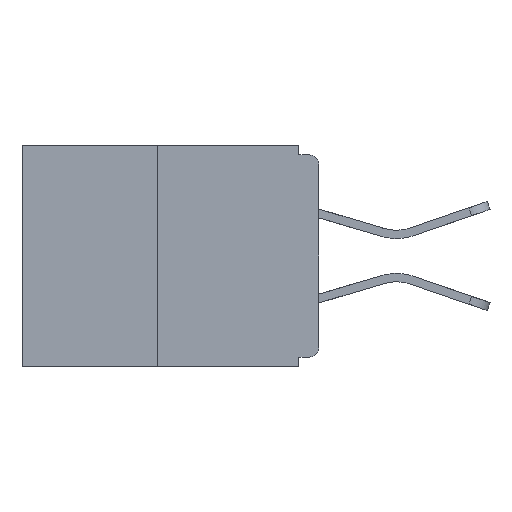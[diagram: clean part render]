
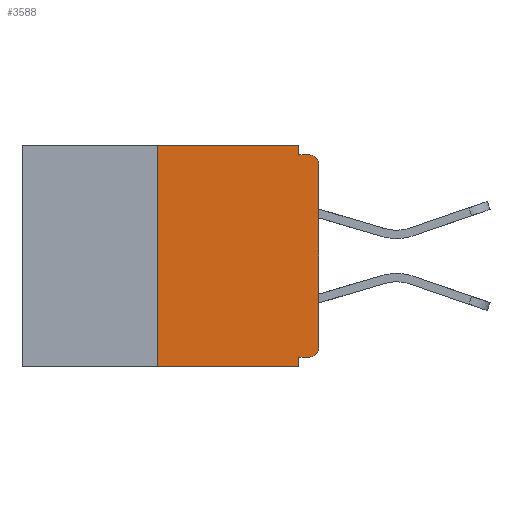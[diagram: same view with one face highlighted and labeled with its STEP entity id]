
A CAD part, left-side view. The second image highlights one B-rep face of the part: STEP entity #3588.
In plain terms, the highlighted planar face has unit normal (-1, 0, 0).
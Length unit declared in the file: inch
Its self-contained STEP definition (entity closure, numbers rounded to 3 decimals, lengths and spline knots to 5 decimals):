
#286 = VERTEX_POINT ( 'NONE', #1986 ) ;
#363 = DIRECTION ( 'NONE',  ( 0., -1., 0. ) ) ;
#559 = CARTESIAN_POINT ( 'NONE',  ( 0., 0.25, 0. ) ) ;
#690 = CARTESIAN_POINT ( 'NONE',  ( 0., 0.46, 0. ) ) ;
#737 = PLANE ( 'NONE',  #10381 ) ;
#957 = ORIENTED_EDGE ( 'NONE', *, *, #11185, .T. ) ;
#1065 = LINE ( 'NONE', #8605, #7907 ) ;
#1281 = CARTESIAN_POINT ( 'NONE',  ( 0., 0.015, -0.015 ) ) ;
#1345 = CARTESIAN_POINT ( 'NONE',  ( 0., 0.015, -0.03 ) ) ;
#1426 = VECTOR ( 'NONE', #13234, 39.37008 ) ;
#1463 = DIRECTION ( 'NONE',  ( 0., -1., 0. ) ) ;
#1663 = LINE ( 'NONE', #2857, #1981 ) ;
#1704 = ORIENTED_EDGE ( 'NONE', *, *, #7658, .T. ) ;
#1903 = VECTOR ( 'NONE', #12912, 39.37008 ) ;
#1948 = CARTESIAN_POINT ( 'NONE',  ( 0., 0., -0.313 ) ) ;
#1981 = VECTOR ( 'NONE', #12138, 39.37008 ) ;
#1986 = CARTESIAN_POINT ( 'NONE',  ( 0., 0.031, -0.015 ) ) ;
#2129 = EDGE_CURVE ( 'NONE', #10455, #8525, #2821, .T. ) ;
#2291 = EDGE_CURVE ( 'NONE', #10760, #11855, #3197, .T. ) ;
#2369 = VERTEX_POINT ( 'NONE', #13059 ) ;
#2490 = ORIENTED_EDGE ( 'NONE', *, *, #3497, .F. ) ;
#2585 = EDGE_LOOP ( 'NONE', ( #2795, #2490, #1704, #7091, #9048, #3241, #957, #9524, #6849, #12381 ) ) ;
#2738 = VERTEX_POINT ( 'NONE', #6238 ) ;
#2795 = ORIENTED_EDGE ( 'NONE', *, *, #9120, .F. ) ;
#2821 = CIRCLE ( 'NONE', #9344, 0.015 ) ;
#2857 = CARTESIAN_POINT ( 'NONE',  ( 0., 0., 0. ) ) ;
#3197 = CIRCLE ( 'NONE', #6318, 0.015 ) ;
#3241 = ORIENTED_EDGE ( 'NONE', *, *, #2291, .T. ) ;
#3264 = EDGE_CURVE ( 'NONE', #2369, #286, #12860, .T. ) ;
#3497 = EDGE_CURVE ( 'NONE', #11511, #11041, #5757, .T. ) ;
#3550 = LINE ( 'NONE', #11971, #1903 ) ;
#3588 = ADVANCED_FACE ( 'NONE', ( #9647 ), #737, .F. ) ;
#3921 = CARTESIAN_POINT ( 'NONE',  ( 0., 0., -0.03 ) ) ;
#3996 = CARTESIAN_POINT ( 'NONE',  ( 0., 0., -0.328 ) ) ;
#4006 = DIRECTION ( 'NONE',  ( 0., 0., -1. ) ) ;
#4123 = VECTOR ( 'NONE', #11197, 39.37008 ) ;
#4186 = DIRECTION ( 'NONE',  ( 0., 0., -1. ) ) ;
#4202 = LINE ( 'NONE', #11248, #1426 ) ;
#4496 = DIRECTION ( 'NONE',  ( -1., 0., 0. ) ) ;
#5285 = CARTESIAN_POINT ( 'NONE',  ( 0., 0.25, -0.343 ) ) ;
#5757 = LINE ( 'NONE', #559, #11089 ) ;
#5895 = DIRECTION ( 'NONE',  ( 0., 0., -1. ) ) ;
#6238 = CARTESIAN_POINT ( 'NONE',  ( 0., 0.031, -0.328 ) ) ;
#6318 = AXIS2_PLACEMENT_3D ( 'NONE', #10951, #9911, #5895 ) ;
#6636 = CARTESIAN_POINT ( 'NONE',  ( 0., 0.031, -0.343 ) ) ;
#6849 = ORIENTED_EDGE ( 'NONE', *, *, #12982, .F. ) ;
#7091 = ORIENTED_EDGE ( 'NONE', *, *, #7758, .F. ) ;
#7441 = DIRECTION ( 'NONE',  ( 0., 0., -1. ) ) ;
#7658 = EDGE_CURVE ( 'NONE', #11511, #11618, #3550, .T. ) ;
#7684 = CARTESIAN_POINT ( 'NONE',  ( 0., 0.25, 0. ) ) ;
#7758 = EDGE_CURVE ( 'NONE', #2738, #11618, #4202, .T. ) ;
#7787 = LINE ( 'NONE', #10745, #8442 ) ;
#7837 = DIRECTION ( 'NONE',  ( 0., 0., 1. ) ) ;
#7907 = VECTOR ( 'NONE', #363, 39.37008 ) ;
#8023 = DIRECTION ( 'NONE',  ( 1., 0., 0. ) ) ;
#8032 = VECTOR ( 'NONE', #4186, 39.37008 ) ;
#8442 = VECTOR ( 'NONE', #1463, 39.37008 ) ;
#8525 = VERTEX_POINT ( 'NONE', #1281 ) ;
#8605 = CARTESIAN_POINT ( 'NONE',  ( 0., 0.46, 0. ) ) ;
#8828 = CARTESIAN_POINT ( 'NONE',  ( 0., 0.015, -0.328 ) ) ;
#9048 = ORIENTED_EDGE ( 'NONE', *, *, #11249, .F. ) ;
#9120 = EDGE_CURVE ( 'NONE', #11041, #2369, #1065, .T. ) ;
#9344 = AXIS2_PLACEMENT_3D ( 'NONE', #1345, #4496, #7441 ) ;
#9524 = ORIENTED_EDGE ( 'NONE', *, *, #2129, .T. ) ;
#9563 = CARTESIAN_POINT ( 'NONE',  ( 0., 0.031, 0. ) ) ;
#9647 = FACE_OUTER_BOUND ( 'NONE', #2585, .T. ) ;
#9911 = DIRECTION ( 'NONE',  ( -1., 0., 0. ) ) ;
#10381 = AXIS2_PLACEMENT_3D ( 'NONE', #690, #8023, #4006 ) ;
#10455 = VERTEX_POINT ( 'NONE', #3921 ) ;
#10745 = CARTESIAN_POINT ( 'NONE',  ( 0., 0., -0.015 ) ) ;
#10760 = VERTEX_POINT ( 'NONE', #8828 ) ;
#10951 = CARTESIAN_POINT ( 'NONE',  ( 0., 0.015, -0.313 ) ) ;
#11041 = VERTEX_POINT ( 'NONE', #7684 ) ;
#11089 = VECTOR ( 'NONE', #7837, 39.37008 ) ;
#11185 = EDGE_CURVE ( 'NONE', #11855, #10455, #1663, .T. ) ;
#11197 = DIRECTION ( 'NONE',  ( 0., 1., 0. ) ) ;
#11217 = LINE ( 'NONE', #3996, #4123 ) ;
#11248 = CARTESIAN_POINT ( 'NONE',  ( 0., 0.031, -0.343 ) ) ;
#11249 = EDGE_CURVE ( 'NONE', #10760, #2738, #11217, .T. ) ;
#11511 = VERTEX_POINT ( 'NONE', #5285 ) ;
#11618 = VERTEX_POINT ( 'NONE', #6636 ) ;
#11855 = VERTEX_POINT ( 'NONE', #1948 ) ;
#11971 = CARTESIAN_POINT ( 'NONE',  ( 0., 0.46, -0.343 ) ) ;
#12138 = DIRECTION ( 'NONE',  ( 0., 0., 1. ) ) ;
#12381 = ORIENTED_EDGE ( 'NONE', *, *, #3264, .F. ) ;
#12860 = LINE ( 'NONE', #9563, #8032 ) ;
#12912 = DIRECTION ( 'NONE',  ( 0., -1., 0. ) ) ;
#12982 = EDGE_CURVE ( 'NONE', #286, #8525, #7787, .T. ) ;
#13059 = CARTESIAN_POINT ( 'NONE',  ( 0., 0.031, 0. ) ) ;
#13234 = DIRECTION ( 'NONE',  ( 0., 0., -1. ) ) ;
